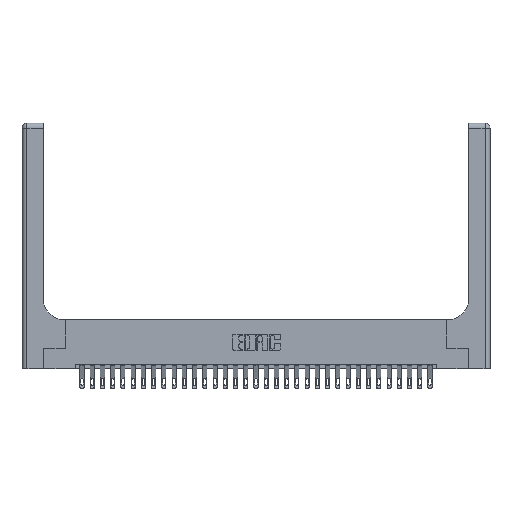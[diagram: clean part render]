
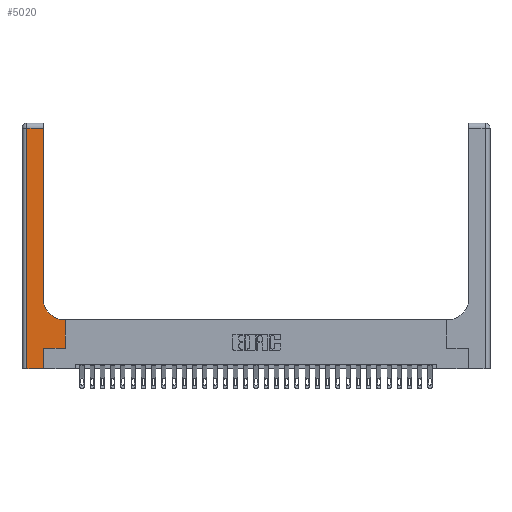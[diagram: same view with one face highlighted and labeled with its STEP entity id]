
A CAD part, top view. The second image highlights one B-rep face of the part: STEP entity #5020.
In plain terms, the highlighted planar face has unit normal (0, 0, 1).
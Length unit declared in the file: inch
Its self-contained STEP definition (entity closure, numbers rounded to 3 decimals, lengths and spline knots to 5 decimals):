
#839 = LINE ( 'NONE', #2442, #17502 ) ;
#1091 = EDGE_CURVE ( 'NONE', #14839, #22022, #12240, .T. ) ;
#1778 = DIRECTION ( 'NONE',  ( 0., 1., 0. ) ) ;
#2074 = ORIENTED_EDGE ( 'NONE', *, *, #26227, .T. ) ;
#2077 = CARTESIAN_POINT ( 'NONE',  ( 0.528, 0.25, 0.37 ) ) ;
#2318 = LINE ( 'NONE', #17219, #29270 ) ;
#2442 = CARTESIAN_POINT ( 'NONE',  ( 0., 2.94, 0.37 ) ) ;
#3622 = LINE ( 'NONE', #14038, #13204 ) ;
#3769 = CARTESIAN_POINT ( 'NONE',  ( 0.06, 2.94, 0.37 ) ) ;
#3829 = DIRECTION ( 'NONE',  ( 0., -1., 0. ) ) ;
#4542 = AXIS2_PLACEMENT_3D ( 'NONE', #17784, #8720, #17684 ) ;
#4849 = VERTEX_POINT ( 'NONE', #16709 ) ;
#4987 = CARTESIAN_POINT ( 'NONE',  ( 0.06, 0., 0.37 ) ) ;
#5020 = ADVANCED_FACE ( 'NONE', ( #16699 ), #15118, .F. ) ;
#5558 = VECTOR ( 'NONE', #22386, 39.37008 ) ;
#5696 = VERTEX_POINT ( 'NONE', #17253 ) ;
#5721 = EDGE_CURVE ( 'NONE', #4849, #14839, #21969, .T. ) ;
#6524 = CARTESIAN_POINT ( 'NONE',  ( 0.528, 0.6, 0.37 ) ) ;
#7682 = EDGE_CURVE ( 'NONE', #22581, #10542, #2318, .T. ) ;
#8720 = DIRECTION ( 'NONE',  ( 0., 0., -1. ) ) ;
#9164 = ORIENTED_EDGE ( 'NONE', *, *, #7682, .T. ) ;
#9733 = EDGE_CURVE ( 'NONE', #22022, #22581, #14316, .T. ) ;
#10542 = VERTEX_POINT ( 'NONE', #28310 ) ;
#11703 = DIRECTION ( 'NONE',  ( 1., 0., 0. ) ) ;
#11906 = LINE ( 'NONE', #13172, #5558 ) ;
#12046 = ORIENTED_EDGE ( 'NONE', *, *, #17933, .T. ) ;
#12199 = DIRECTION ( 'NONE',  ( -1., 0., 0. ) ) ;
#12222 = VERTEX_POINT ( 'NONE', #3769 ) ;
#12240 = LINE ( 'NONE', #16928, #14328 ) ;
#12244 = ORIENTED_EDGE ( 'NONE', *, *, #18507, .T. ) ;
#13057 = DIRECTION ( 'NONE',  ( 0., 1., 0. ) ) ;
#13172 = CARTESIAN_POINT ( 'NONE',  ( 0.265, 0., 0.37 ) ) ;
#13204 = VECTOR ( 'NONE', #11703, 39.37008 ) ;
#13992 = ORIENTED_EDGE ( 'NONE', *, *, #9733, .T. ) ;
#14038 = CARTESIAN_POINT ( 'NONE',  ( 0.265, 0.25, 0.37 ) ) ;
#14069 = CARTESIAN_POINT ( 'NONE',  ( 0., 0., 0.37 ) ) ;
#14316 = CIRCLE ( 'NONE', #15434, 0.25 ) ;
#14328 = VECTOR ( 'NONE', #12199, 39.37008 ) ;
#14443 = CARTESIAN_POINT ( 'NONE',  ( 0.26, 0.85, 0.37 ) ) ;
#14584 = CARTESIAN_POINT ( 'NONE',  ( 0.51, 0.6, 0.37 ) ) ;
#14839 = VERTEX_POINT ( 'NONE', #6524 ) ;
#14931 = VERTEX_POINT ( 'NONE', #22817 ) ;
#15118 = PLANE ( 'NONE',  #4542 ) ;
#15434 = AXIS2_PLACEMENT_3D ( 'NONE', #15794, #27143, #27640 ) ;
#15575 = EDGE_CURVE ( 'NONE', #23056, #5696, #26533, .T. ) ;
#15794 = CARTESIAN_POINT ( 'NONE',  ( 0.51, 0.85, 0.37 ) ) ;
#15979 = VECTOR ( 'NONE', #1778, 39.37008 ) ;
#16699 = FACE_OUTER_BOUND ( 'NONE', #22688, .T. ) ;
#16709 = CARTESIAN_POINT ( 'NONE',  ( 0.528, 0.25, 0.37 ) ) ;
#16928 = CARTESIAN_POINT ( 'NONE',  ( 0.26, 0.6, 0.37 ) ) ;
#17219 = CARTESIAN_POINT ( 'NONE',  ( 0.26, 3., 0.37 ) ) ;
#17253 = CARTESIAN_POINT ( 'NONE',  ( 0.265, 0., 0.37 ) ) ;
#17502 = VECTOR ( 'NONE', #18231, 39.37008 ) ;
#17684 = DIRECTION ( 'NONE',  ( -1., 0., 0. ) ) ;
#17784 = CARTESIAN_POINT ( 'NONE',  ( 0., 3., 0.37 ) ) ;
#17933 = EDGE_CURVE ( 'NONE', #5696, #14931, #11906, .T. ) ;
#18079 = VECTOR ( 'NONE', #23079, 39.37008 ) ;
#18231 = DIRECTION ( 'NONE',  ( -1., 0., 0. ) ) ;
#18507 = EDGE_CURVE ( 'NONE', #12222, #23056, #22139, .T. ) ;
#18980 = VECTOR ( 'NONE', #3829, 39.37008 ) ;
#20315 = ORIENTED_EDGE ( 'NONE', *, *, #1091, .T. ) ;
#20508 = ORIENTED_EDGE ( 'NONE', *, *, #15575, .T. ) ;
#21969 = LINE ( 'NONE', #2077, #15979 ) ;
#22022 = VERTEX_POINT ( 'NONE', #14584 ) ;
#22139 = LINE ( 'NONE', #24305, #18980 ) ;
#22386 = DIRECTION ( 'NONE',  ( 0., 1., 0. ) ) ;
#22581 = VERTEX_POINT ( 'NONE', #14443 ) ;
#22688 = EDGE_LOOP ( 'NONE', ( #9164, #24627, #12244, #20508, #12046, #2074, #24893, #20315, #13992 ) ) ;
#22817 = CARTESIAN_POINT ( 'NONE',  ( 0.265, 0.25, 0.37 ) ) ;
#23056 = VERTEX_POINT ( 'NONE', #4987 ) ;
#23079 = DIRECTION ( 'NONE',  ( 1., 0., 0. ) ) ;
#24305 = CARTESIAN_POINT ( 'NONE',  ( 0.06, 3., 0.37 ) ) ;
#24627 = ORIENTED_EDGE ( 'NONE', *, *, #25458, .T. ) ;
#24893 = ORIENTED_EDGE ( 'NONE', *, *, #5721, .T. ) ;
#25458 = EDGE_CURVE ( 'NONE', #10542, #12222, #839, .T. ) ;
#26227 = EDGE_CURVE ( 'NONE', #14931, #4849, #3622, .T. ) ;
#26533 = LINE ( 'NONE', #14069, #18079 ) ;
#27143 = DIRECTION ( 'NONE',  ( 0., 0., -1. ) ) ;
#27640 = DIRECTION ( 'NONE',  ( 1., 0., 0. ) ) ;
#28310 = CARTESIAN_POINT ( 'NONE',  ( 0.26, 2.94, 0.37 ) ) ;
#29270 = VECTOR ( 'NONE', #13057, 39.37008 ) ;
